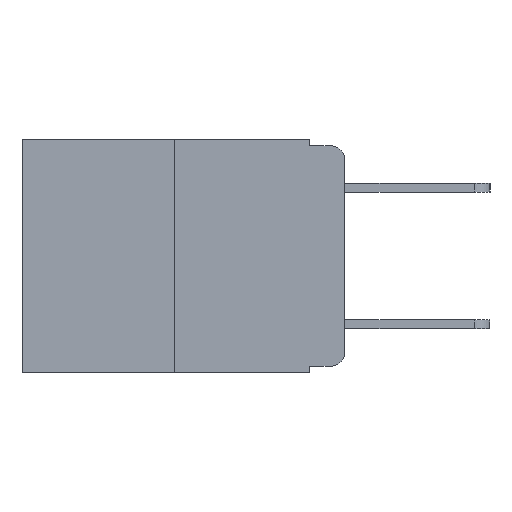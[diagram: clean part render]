
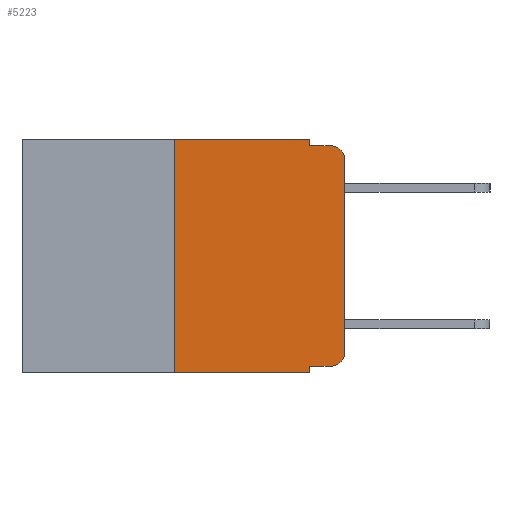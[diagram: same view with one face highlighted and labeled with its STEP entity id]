
A CAD part, left-side view. The second image highlights one B-rep face of the part: STEP entity #5223.
In plain terms, the highlighted planar face has unit normal (-1, 0, 0).
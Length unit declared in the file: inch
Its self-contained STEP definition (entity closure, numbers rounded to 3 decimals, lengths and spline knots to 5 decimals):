
#295 = VECTOR ( 'NONE', #9114, 39.37008 ) ;
#304 = DIRECTION ( 'NONE',  ( 0., 0., -1. ) ) ;
#356 = CARTESIAN_POINT ( 'NONE',  ( 0., 0.25, 0. ) ) ;
#495 = CARTESIAN_POINT ( 'NONE',  ( 0., 0.051, 0. ) ) ;
#687 = DIRECTION ( 'NONE',  ( -1., 0., 0. ) ) ;
#920 = CARTESIAN_POINT ( 'NONE',  ( 0., 0.051, 0. ) ) ;
#926 = CARTESIAN_POINT ( 'NONE',  ( 0., 0.051, -0.01 ) ) ;
#953 = EDGE_CURVE ( 'NONE', #9444, #3371, #6129, .T. ) ;
#989 = VERTEX_POINT ( 'NONE', #356 ) ;
#993 = CIRCLE ( 'NONE', #1164, 0.02 ) ;
#1011 = VERTEX_POINT ( 'NONE', #926 ) ;
#1040 = EDGE_CURVE ( 'NONE', #5349, #1011, #5601, .T. ) ;
#1065 = CARTESIAN_POINT ( 'NONE',  ( 0., 0.02, -0.01 ) ) ;
#1164 = AXIS2_PLACEMENT_3D ( 'NONE', #7983, #3055, #8765 ) ;
#1283 = DIRECTION ( 'NONE',  ( 0., 0., -1. ) ) ;
#1716 = CARTESIAN_POINT ( 'NONE',  ( 0., 0.25, -0.343 ) ) ;
#1913 = CARTESIAN_POINT ( 'NONE',  ( 0., 0.02, -0.333 ) ) ;
#2174 = CARTESIAN_POINT ( 'NONE',  ( 0., 0.051, -0.333 ) ) ;
#2335 = EDGE_CURVE ( 'NONE', #9444, #6639, #6221, .T. ) ;
#2420 = VERTEX_POINT ( 'NONE', #1716 ) ;
#2453 = CIRCLE ( 'NONE', #7638, 0.02 ) ;
#2472 = LINE ( 'NONE', #9525, #10576 ) ;
#2564 = VECTOR ( 'NONE', #7802, 39.37008 ) ;
#2572 = CARTESIAN_POINT ( 'NONE',  ( 0., 0.051, 0. ) ) ;
#2696 = DIRECTION ( 'NONE',  ( 0., -1., 0. ) ) ;
#2850 = CARTESIAN_POINT ( 'NONE',  ( 0., 0.473, -0.343 ) ) ;
#3055 = DIRECTION ( 'NONE',  ( -1., 0., 0. ) ) ;
#3371 = VERTEX_POINT ( 'NONE', #3402 ) ;
#3401 = CARTESIAN_POINT ( 'NONE',  ( 0., 0.051, -0.01 ) ) ;
#3402 = CARTESIAN_POINT ( 'NONE',  ( 0., 0.051, -0.343 ) ) ;
#3494 = ORIENTED_EDGE ( 'NONE', *, *, #10608, .T. ) ;
#3523 = ORIENTED_EDGE ( 'NONE', *, *, #8350, .T. ) ;
#3535 = ORIENTED_EDGE ( 'NONE', *, *, #8142, .F. ) ;
#3576 = ORIENTED_EDGE ( 'NONE', *, *, #1040, .F. ) ;
#3590 = ORIENTED_EDGE ( 'NONE', *, *, #8976, .F. ) ;
#3649 = ORIENTED_EDGE ( 'NONE', *, *, #7049, .F. ) ;
#3671 = ORIENTED_EDGE ( 'NONE', *, *, #5467, .T. ) ;
#3688 = ORIENTED_EDGE ( 'NONE', *, *, #953, .F. ) ;
#3699 = ORIENTED_EDGE ( 'NONE', *, *, #2335, .T. ) ;
#3733 = ORIENTED_EDGE ( 'NONE', *, *, #8054, .T. ) ;
#3895 = VECTOR ( 'NONE', #7529, 39.37008 ) ;
#4129 = LINE ( 'NONE', #2850, #8398 ) ;
#4979 = DIRECTION ( 'NONE',  ( 0., 0., 1. ) ) ;
#5168 = FACE_OUTER_BOUND ( 'NONE', #5314, .T. ) ;
#5223 = ADVANCED_FACE ( 'NONE', ( #5168 ), #6032, .F. ) ;
#5314 = EDGE_LOOP ( 'NONE', ( #3494, #3523, #3535, #3576, #3590, #3649, #3671, #3688, #3699, #3733 ) ) ;
#5349 = VERTEX_POINT ( 'NONE', #2572 ) ;
#5467 = EDGE_CURVE ( 'NONE', #2420, #3371, #4129, .T. ) ;
#5601 = LINE ( 'NONE', #920, #9373 ) ;
#6013 = CARTESIAN_POINT ( 'NONE',  ( 0., 0.02, -0.313 ) ) ;
#6032 = PLANE ( 'NONE',  #8263 ) ;
#6092 = DIRECTION ( 'NONE',  ( 0., 0., -1. ) ) ;
#6117 = VERTEX_POINT ( 'NONE', #8076 ) ;
#6129 = LINE ( 'NONE', #495, #9802 ) ;
#6221 = LINE ( 'NONE', #2174, #9870 ) ;
#6639 = VERTEX_POINT ( 'NONE', #1913 ) ;
#6802 = DIRECTION ( 'NONE',  ( 0., 0., -1. ) ) ;
#6877 = VERTEX_POINT ( 'NONE', #7204 ) ;
#7049 = EDGE_CURVE ( 'NONE', #2420, #989, #2472, .T. ) ;
#7089 = CARTESIAN_POINT ( 'NONE',  ( 0., 0.473, 0. ) ) ;
#7204 = CARTESIAN_POINT ( 'NONE',  ( 0., 0., -0.313 ) ) ;
#7288 = LINE ( 'NONE', #8365, #295 ) ;
#7529 = DIRECTION ( 'NONE',  ( 0., -1., 0. ) ) ;
#7638 = AXIS2_PLACEMENT_3D ( 'NONE', #6013, #687, #6802 ) ;
#7802 = DIRECTION ( 'NONE',  ( 0., -1., 0. ) ) ;
#7983 = CARTESIAN_POINT ( 'NONE',  ( 0., 0.02, -0.03 ) ) ;
#8054 = EDGE_CURVE ( 'NONE', #6639, #6877, #2453, .T. ) ;
#8076 = CARTESIAN_POINT ( 'NONE',  ( 0., 0., -0.03 ) ) ;
#8142 = EDGE_CURVE ( 'NONE', #1011, #10066, #8211, .T. ) ;
#8211 = LINE ( 'NONE', #3401, #3895 ) ;
#8263 = AXIS2_PLACEMENT_3D ( 'NONE', #8813, #9619, #6092 ) ;
#8350 = EDGE_CURVE ( 'NONE', #6117, #10066, #993, .T. ) ;
#8365 = CARTESIAN_POINT ( 'NONE',  ( 0., 0., 0. ) ) ;
#8398 = VECTOR ( 'NONE', #8473, 39.37008 ) ;
#8473 = DIRECTION ( 'NONE',  ( 0., -1., 0. ) ) ;
#8765 = DIRECTION ( 'NONE',  ( 0., 0., -1. ) ) ;
#8813 = CARTESIAN_POINT ( 'NONE',  ( 0., 0.473, 0. ) ) ;
#8976 = EDGE_CURVE ( 'NONE', #989, #5349, #10225, .T. ) ;
#9114 = DIRECTION ( 'NONE',  ( 0., 0., 1. ) ) ;
#9373 = VECTOR ( 'NONE', #304, 39.37008 ) ;
#9444 = VERTEX_POINT ( 'NONE', #9778 ) ;
#9525 = CARTESIAN_POINT ( 'NONE',  ( 0., 0.25, 0. ) ) ;
#9619 = DIRECTION ( 'NONE',  ( 1., 0., 0. ) ) ;
#9778 = CARTESIAN_POINT ( 'NONE',  ( 0., 0.051, -0.333 ) ) ;
#9802 = VECTOR ( 'NONE', #1283, 39.37008 ) ;
#9870 = VECTOR ( 'NONE', #2696, 39.37008 ) ;
#10066 = VERTEX_POINT ( 'NONE', #1065 ) ;
#10225 = LINE ( 'NONE', #7089, #2564 ) ;
#10576 = VECTOR ( 'NONE', #4979, 39.37008 ) ;
#10608 = EDGE_CURVE ( 'NONE', #6877, #6117, #7288, .T. ) ;
